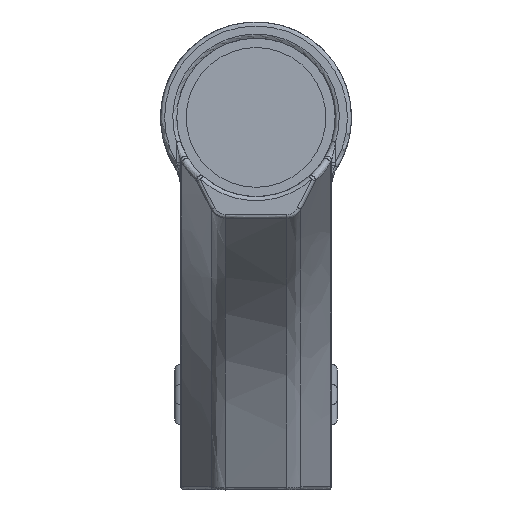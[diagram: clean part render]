
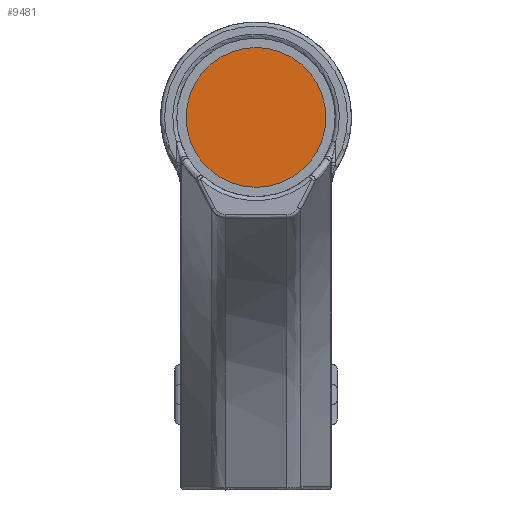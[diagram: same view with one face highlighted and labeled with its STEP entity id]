
A CAD part, front view. The second image highlights one B-rep face of the part: STEP entity #9481.
In plain terms, the highlighted planar face has unit normal (0, -1, 0).
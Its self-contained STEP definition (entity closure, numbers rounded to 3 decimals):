
#886=CIRCLE('',#10316,17.2);
#1083=PLANE('',#10315);
#1568=FACE_OUTER_BOUND('',#2137,.T.);
#2137=EDGE_LOOP('',(#8580));
#4505=VERTEX_POINT('',#21582);
#5891=EDGE_CURVE('',#4505,#4505,#886,.T.);
#8580=ORIENTED_EDGE('',*,*,#5891,.T.);
#9481=ADVANCED_FACE('',(#1568),#1083,.F.);
#10315=AXIS2_PLACEMENT_3D('',#21581,#12579,#12580);
#10316=AXIS2_PLACEMENT_3D('',#21583,#12581,#12582);
#12579=DIRECTION('center_axis',(0.,1.,0.));
#12580=DIRECTION('ref_axis',(-1.,0.,0.));
#12581=DIRECTION('center_axis',(0.,-1.,0.));
#12582=DIRECTION('ref_axis',(0.,0.,
1.));
#21581=CARTESIAN_POINT('Origin',(19.128,66.521,83.783));
#21582=CARTESIAN_POINT('',(19.128,66.521,100.983));
#21583=CARTESIAN_POINT('Origin',(19.128,66.521,83.783));
